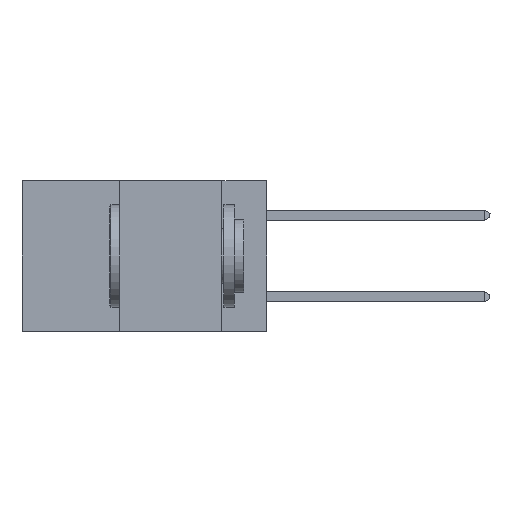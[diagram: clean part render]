
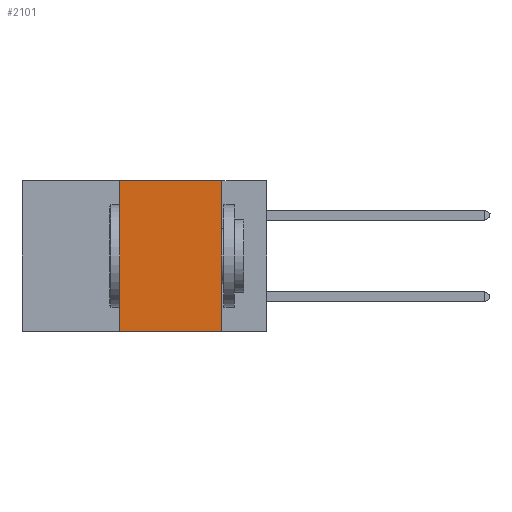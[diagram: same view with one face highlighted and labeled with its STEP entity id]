
A CAD part, left-side view. The second image highlights one B-rep face of the part: STEP entity #2101.
In plain terms, the highlighted planar face has unit normal (-1, 0, 0).
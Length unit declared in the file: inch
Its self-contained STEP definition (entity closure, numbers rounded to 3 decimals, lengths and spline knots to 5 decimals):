
#19 = CARTESIAN_POINT ( 'NONE',  ( 0., 0.11, 0. ) ) ;
#384 = VECTOR ( 'NONE', #16546, 39.37008 ) ;
#1536 = LINE ( 'NONE', #5477, #7426 ) ;
#1667 = EDGE_CURVE ( 'NONE', #21210, #21127, #13426, .T. ) ;
#2101 = ADVANCED_FACE ( 'NONE', ( #6030 ), #9701, .F. ) ;
#2169 = LINE ( 'NONE', #17907, #12055 ) ;
#5477 = CARTESIAN_POINT ( 'NONE',  ( 0., 0.6, 0. ) ) ;
#6030 = FACE_OUTER_BOUND ( 'NONE', #23588, .T. ) ;
#6517 = ORIENTED_EDGE ( 'NONE', *, *, #11855, .F. ) ;
#7377 = DIRECTION ( 'NONE',  ( 0., -1., 0. ) ) ;
#7426 = VECTOR ( 'NONE', #7377, 39.37008 ) ;
#9013 = ORIENTED_EDGE ( 'NONE', *, *, #21716, .F. ) ;
#9701 = PLANE ( 'NONE',  #18454 ) ;
#11707 = VERTEX_POINT ( 'NONE', #15168 ) ;
#11855 = EDGE_CURVE ( 'NONE', #11707, #21127, #15231, .T. ) ;
#12055 = VECTOR ( 'NONE', #17998, 39.37008 ) ;
#12687 = EDGE_CURVE ( 'NONE', #21210, #17933, #2169, .T. ) ;
#13145 = ORIENTED_EDGE ( 'NONE', *, *, #1667, .T. ) ;
#13426 = LINE ( 'NONE', #22323, #384 ) ;
#13476 = CARTESIAN_POINT ( 'NONE',  ( 0., 0.36, -0.37 ) ) ;
#14627 = VECTOR ( 'NONE', #15835, 39.37008 ) ;
#15168 = CARTESIAN_POINT ( 'NONE',  ( 0., 0.11, 0. ) ) ;
#15231 = LINE ( 'NONE', #19, #14627 ) ;
#15463 = DIRECTION ( 'NONE',  ( 0., 0., -1. ) ) ;
#15835 = DIRECTION ( 'NONE',  ( 0., 0., -1. ) ) ;
#16546 = DIRECTION ( 'NONE',  ( 0., -1., 0. ) ) ;
#17504 = CARTESIAN_POINT ( 'NONE',  ( 0., 0.6, 0. ) ) ;
#17907 = CARTESIAN_POINT ( 'NONE',  ( 0., 0.36, 0. ) ) ;
#17933 = VERTEX_POINT ( 'NONE', #18221 ) ;
#17998 = DIRECTION ( 'NONE',  ( 0., 0., 1. ) ) ;
#18221 = CARTESIAN_POINT ( 'NONE',  ( 0., 0.36, 0. ) ) ;
#18454 = AXIS2_PLACEMENT_3D ( 'NONE', #17504, #21847, #15463 ) ;
#20943 = ORIENTED_EDGE ( 'NONE', *, *, #12687, .F. ) ;
#21127 = VERTEX_POINT ( 'NONE', #23019 ) ;
#21210 = VERTEX_POINT ( 'NONE', #13476 ) ;
#21716 = EDGE_CURVE ( 'NONE', #17933, #11707, #1536, .T. ) ;
#21847 = DIRECTION ( 'NONE',  ( 1., 0., 0. ) ) ;
#22323 = CARTESIAN_POINT ( 'NONE',  ( 0., 0.6, -0.37 ) ) ;
#23019 = CARTESIAN_POINT ( 'NONE',  ( 0., 0.11, -0.37 ) ) ;
#23588 = EDGE_LOOP ( 'NONE', ( #6517, #9013, #20943, #13145 ) ) ;
